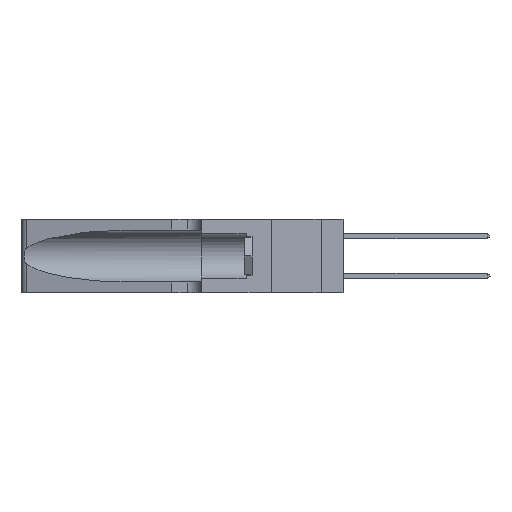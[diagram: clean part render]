
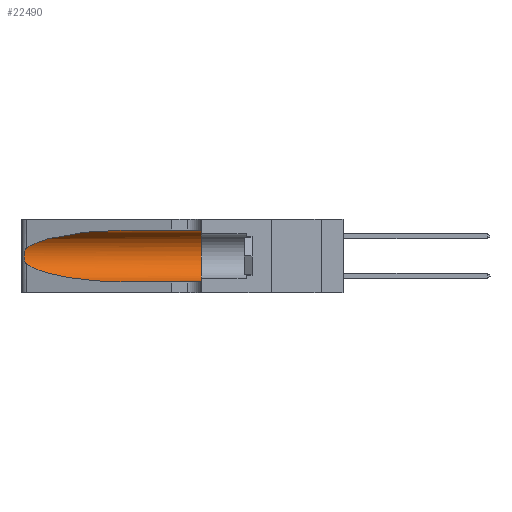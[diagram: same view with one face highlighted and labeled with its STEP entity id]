
A CAD part, left-side view. The second image highlights one B-rep face of the part: STEP entity #22490.
In plain terms, the highlighted cylindrical face has radius 3.308 mm (diameter 6.617 mm), a partial arc.
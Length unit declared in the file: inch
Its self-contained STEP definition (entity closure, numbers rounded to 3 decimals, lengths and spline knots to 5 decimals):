
#1416 = EDGE_LOOP ( 'NONE', ( #19633, #8807, #28630, #37070, #42890, #18590 ) ) ;
#3241 = CARTESIAN_POINT ( 'NONE',  ( 0.25487, 1.22718, 0.22369 ) ) ;
#5895 = CARTESIAN_POINT ( 'NONE',  ( 0.25487, 1.22718, 0.14631 ) ) ;
#6995 = DIRECTION ( 'NONE',  ( 0., 0., -1. ) ) ;
#7300 = CARTESIAN_POINT ( 'NONE',  ( 0.25555, 1.22993, 0.14849 ) ) ;
#7460 = CARTESIAN_POINT ( 'NONE',  ( 0.26018, 1.23835, 0.19895 ) ) ;
#7748 = CARTESIAN_POINT ( 'NONE',  ( 0.25854, 1.2359, 0.20912 ) ) ;
#7759 = CARTESIAN_POINT ( 'NONE',  ( 0.1305, 0.72297, 0.05475 ) ) ;
#8807 = ORIENTED_EDGE ( 'NONE', *, *, #39865, .T. ) ;
#9192 = VECTOR ( 'NONE', #34087, 39.37008 ) ;
#9401 = CARTESIAN_POINT ( 'NONE',  ( 0.25487, 1.22718, 0.22369 ) ) ;
#9893 = VECTOR ( 'NONE', #25478, 39.37008 ) ;
#10238 = VERTEX_POINT ( 'NONE', #3241 ) ;
#10731 = FACE_OUTER_BOUND ( 'NONE', #1416, .T. ) ;
#10802 = CARTESIAN_POINT ( 'NONE',  ( 0.25789, 1.23486, 0.15765 ) ) ;
#11096 = CARTESIAN_POINT ( 'NONE',  ( 0.25856, 1.23593, 0.16098 ) ) ;
#11389 = CARTESIAN_POINT ( 'NONE',  ( 0.25487, 1.22718, 0.14631 ) ) ;
#12112 = CARTESIAN_POINT ( 'NONE',  ( 0.18966, 0.96281, 0.31525 ) ) ;
#13174 = CARTESIAN_POINT ( 'NONE',  ( 0.2373, 1.15595, 0.28018 ) ) ;
#13688 = DIRECTION ( 'NONE',  ( 0., -1., 0. ) ) ;
#14516 = VERTEX_POINT ( 'NONE', #25780 ) ;
#14591 = CARTESIAN_POINT ( 'NONE',  ( 0.25639, 1.23186, 0.15144 ) ) ;
#15964 = EDGE_CURVE ( 'NONE', #21527, #29856, #42542, .T. ) ;
#16343 = CARTESIAN_POINT ( 'NONE',  ( 0.2373, 1.15595, 0.08982 ) ) ;
#17889 =( BOUNDED_CURVE ( )  B_SPLINE_CURVE ( 3, ( #33588, #16343, #40543, #33744 ),
 .UNSPECIFIED., .F., .F. ) 
 B_SPLINE_CURVE_WITH_KNOTS ( ( 4, 4 ),
 ( 3.44316, 4.71239 ),
 .UNSPECIFIED. ) 
 CURVE ( )  GEOMETRIC_REPRESENTATION_ITEM ( )  RATIONAL_B_SPLINE_CURVE ( ( 1., 0.87, 0.87, 1. ) ) 
 REPRESENTATION_ITEM ( '' )  );
#17917 = CARTESIAN_POINT ( 'NONE',  ( 0.26075, 1.23896, 0.19203 ) ) ;
#18210 = CARTESIAN_POINT ( 'NONE',  ( 0.25487, 1.22718, 0.22369 ) ) ;
#18283 = CARTESIAN_POINT ( 'NONE',  ( 0.1305, 0.35, 0.31525 ) ) ;
#18590 = ORIENTED_EDGE ( 'NONE', *, *, #42187, .F. ) ;
#18703 = EDGE_CURVE ( 'NONE', #33930, #41789, #17889, .T. ) ;
#18931 = CARTESIAN_POINT ( 'NONE',  ( 0.1305, 0.72297, 0.31525 ) ) ;
#19091 = LINE ( 'NONE', #25783, #9893 ) ;
#19633 = ORIENTED_EDGE ( 'NONE', *, *, #33843, .T. ) ;
#21527 = VERTEX_POINT ( 'NONE', #18283 ) ;
#22490 = ADVANCED_FACE ( 'NONE', ( #10731 ), #44307, .F. ) ;
#22847 = AXIS2_PLACEMENT_3D ( 'NONE', #44710, #13688, #6995 ) ;
#22924 = DIRECTION ( 'NONE',  ( 0., 0., 1. ) ) ;
#23268 = LINE ( 'NONE', #44088, #9192 ) ;
#23993 = B_SPLINE_CURVE_WITH_KNOTS ( 'NONE', 3,
 ( #18210, #39103, #31679, #38950, #7748, #7460, #17917, #28214, #28064, #11096, #10802, #14591, #7300, #11389 ),
 .UNSPECIFIED., .F., .F.,
 ( 4, 2, 2, 2, 2, 2, 4 ),
 ( 0., 0.00027, 0.00053, 0.00107, 0.0016, 0.00187, 0.00214 ),
 .UNSPECIFIED. ) ;
#25478 = DIRECTION ( 'NONE',  ( 0., -1., 0. ) ) ;
#25780 = CARTESIAN_POINT ( 'NONE',  ( 0.1305, 0.72297, 0.31525 ) ) ;
#25783 = CARTESIAN_POINT ( 'NONE',  ( 0.1305, 1.61858, 0.05475 ) ) ;
#28064 = CARTESIAN_POINT ( 'NONE',  ( 0.26017, 1.23833, 0.17102 ) ) ;
#28214 = CARTESIAN_POINT ( 'NONE',  ( 0.26075, 1.23896, 0.178 ) ) ;
#28630 = ORIENTED_EDGE ( 'NONE', *, *, #18703, .T. ) ;
#29856 = VERTEX_POINT ( 'NONE', #43716 ) ;
#31679 = CARTESIAN_POINT ( 'NONE',  ( 0.25639, 1.23184, 0.21858 ) ) ;
#33352 = DIRECTION ( 'NONE',  ( 0., 1., 0. ) ) ;
#33588 = CARTESIAN_POINT ( 'NONE',  ( 0.25487, 1.22718, 0.14631 ) ) ;
#33744 = CARTESIAN_POINT ( 'NONE',  ( 0.1305, 0.72297, 0.05475 ) ) ;
#33843 = EDGE_CURVE ( 'NONE', #14516, #10238, #38132, .T. ) ;
#33930 = VERTEX_POINT ( 'NONE', #5895 ) ;
#34087 = DIRECTION ( 'NONE',  ( 0., -1., 0. ) ) ;
#37070 = ORIENTED_EDGE ( 'NONE', *, *, #40636, .T. ) ;
#38132 =( BOUNDED_CURVE ( )  B_SPLINE_CURVE ( 3, ( #18931, #12112, #13174, #9401 ),
 .UNSPECIFIED., .F., .T. ) 
 B_SPLINE_CURVE_WITH_KNOTS ( ( 4, 4 ),
 ( 1.5708, 2.84003 ),
 .UNSPECIFIED. ) 
 CURVE ( )  GEOMETRIC_REPRESENTATION_ITEM ( )  RATIONAL_B_SPLINE_CURVE ( ( 1., 0.87, 0.87, 1. ) ) 
 REPRESENTATION_ITEM ( '' )  );
#38950 = CARTESIAN_POINT ( 'NONE',  ( 0.25787, 1.23484, 0.2124 ) ) ;
#39103 = CARTESIAN_POINT ( 'NONE',  ( 0.25555, 1.22994, 0.2215 ) ) ;
#39865 = EDGE_CURVE ( 'NONE', #10238, #33930, #23993, .T. ) ;
#40543 = CARTESIAN_POINT ( 'NONE',  ( 0.18966, 0.96281, 0.05475 ) ) ;
#40636 = EDGE_CURVE ( 'NONE', #41789, #29856, #19091, .T. ) ;
#40928 = AXIS2_PLACEMENT_3D ( 'NONE', #44109, #33352, #22924 ) ;
#41789 = VERTEX_POINT ( 'NONE', #7759 ) ;
#42187 = EDGE_CURVE ( 'NONE', #14516, #21527, #23268, .T. ) ;
#42542 = CIRCLE ( 'NONE', #40928, 0.13025 ) ;
#42890 = ORIENTED_EDGE ( 'NONE', *, *, #15964, .F. ) ;
#43716 = CARTESIAN_POINT ( 'NONE',  ( 0.1305, 0.35, 0.05475 ) ) ;
#44088 = CARTESIAN_POINT ( 'NONE',  ( 0.1305, 1.61858, 0.31525 ) ) ;
#44109 = CARTESIAN_POINT ( 'NONE',  ( 0.1305, 0.35, 0.185 ) ) ;
#44307 = CYLINDRICAL_SURFACE ( 'NONE', #22847, 0.13025 ) ;
#44710 = CARTESIAN_POINT ( 'NONE',  ( 0.1305, 1.61858, 0.185 ) ) ;
